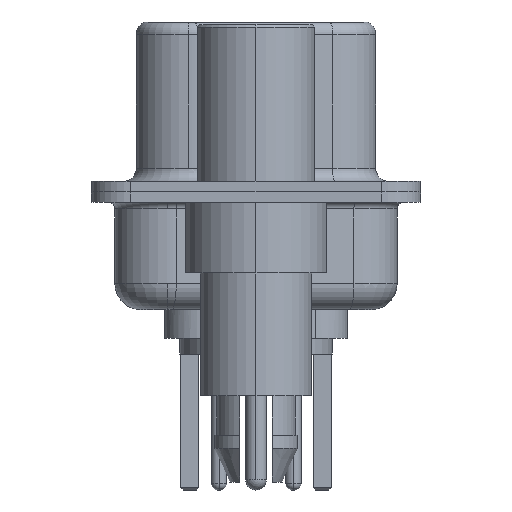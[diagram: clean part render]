
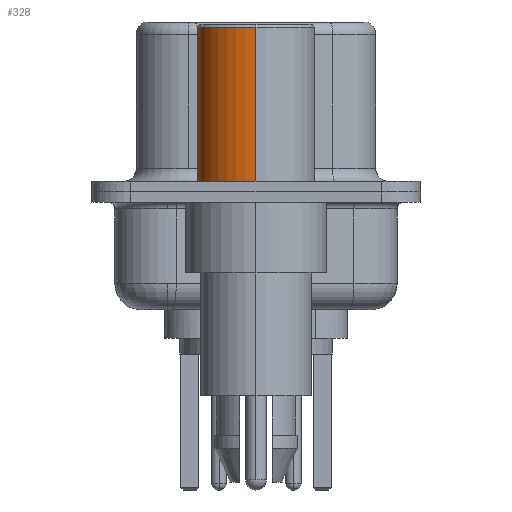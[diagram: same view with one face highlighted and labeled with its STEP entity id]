
A CAD part, left-side view. The second image highlights one B-rep face of the part: STEP entity #328.
In plain terms, the highlighted cylindrical face has radius 2.25 mm (diameter 4.5 mm), a partial arc.
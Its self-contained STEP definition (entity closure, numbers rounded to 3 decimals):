
#328 = ADVANCED_FACE ( 'NONE', ( #14448 ), #23224, .T. ) ;
#1615 = LINE ( 'NONE', #18376, #10739 ) ;
#1768 = DIRECTION ( 'NONE',  ( 0., 0., 1. ) ) ;
#2611 = EDGE_LOOP ( 'NONE', ( #22051, #18080, #4551, #18204 ) ) ;
#4551 = ORIENTED_EDGE ( 'NONE', *, *, #12915, .F. ) ;
#6373 = DIRECTION ( 'NONE',  ( 0., 0., 1. ) ) ;
#7172 = AXIS2_PLACEMENT_3D ( 'NONE', #18447, #7749, #20187 ) ;
#7403 = CARTESIAN_POINT ( 'NONE',  ( 2.25, 0., 6.3 ) ) ;
#7749 = DIRECTION ( 'NONE',  ( 0., 0., 1. ) ) ;
#8618 = DIRECTION ( 'NONE',  ( 0., 0., 1. ) ) ;
#8776 = DIRECTION ( 'NONE',  ( 1., 0., 0. ) ) ;
#8782 = VECTOR ( 'NONE', #1768, 1000. ) ;
#9493 = DIRECTION ( 'NONE',  ( 0., 0., 1. ) ) ;
#10023 = CARTESIAN_POINT ( 'NONE',  ( -2.25, 0., 6.3 ) ) ;
#10739 = VECTOR ( 'NONE', #9493, 1000. ) ;
#11280 = CIRCLE ( 'NONE', #7172, 2.25 ) ;
#11945 = AXIS2_PLACEMENT_3D ( 'NONE', #17045, #6373, #18809 ) ;
#12599 = EDGE_CURVE ( 'NONE', #22747, #16865, #18268, .T. ) ;
#12715 = CIRCLE ( 'NONE', #11945, 2.25 ) ;
#12765 = EDGE_CURVE ( 'NONE', #21992, #21945, #1615, .T. ) ;
#12803 = EDGE_CURVE ( 'NONE', #22747, #21992, #11280, .T. ) ;
#12915 = EDGE_CURVE ( 'NONE', #16865, #21945, #12715, .T. ) ;
#14272 = CARTESIAN_POINT ( 'NONE',  ( 0., 0., 0.581 ) ) ;
#14448 = FACE_OUTER_BOUND ( 'NONE', #2611, .T. ) ;
#14470 = CARTESIAN_POINT ( 'NONE',  ( 2.25, 0., 0.581 ) ) ;
#16865 = VERTEX_POINT ( 'NONE', #7403 ) ;
#17045 = CARTESIAN_POINT ( 'NONE',  ( 0., 0., 6.3 ) ) ;
#18080 = ORIENTED_EDGE ( 'NONE', *, *, #12765, .T. ) ;
#18204 = ORIENTED_EDGE ( 'NONE', *, *, #12599, .F. ) ;
#18268 = LINE ( 'NONE', #14470, #8782 ) ;
#18376 = CARTESIAN_POINT ( 'NONE',  ( -2.25, 0., 0.581 ) ) ;
#18447 = CARTESIAN_POINT ( 'NONE',  ( 0., 0., 0.4 ) ) ;
#18547 = AXIS2_PLACEMENT_3D ( 'NONE', #14272, #8618, #8776 ) ;
#18809 = DIRECTION ( 'NONE',  ( 1., 0., 0. ) ) ;
#19041 = CARTESIAN_POINT ( 'NONE',  ( -2.25, 0., 0.4 ) ) ;
#19246 = CARTESIAN_POINT ( 'NONE',  ( 2.25, 0., 0.4 ) ) ;
#20187 = DIRECTION ( 'NONE',  ( 1., 0., 0. ) ) ;
#21945 = VERTEX_POINT ( 'NONE', #10023 ) ;
#21992 = VERTEX_POINT ( 'NONE', #19041 ) ;
#22051 = ORIENTED_EDGE ( 'NONE', *, *, #12803, .T. ) ;
#22747 = VERTEX_POINT ( 'NONE', #19246 ) ;
#23224 = CYLINDRICAL_SURFACE ( 'NONE', #18547, 2.25 ) ;
